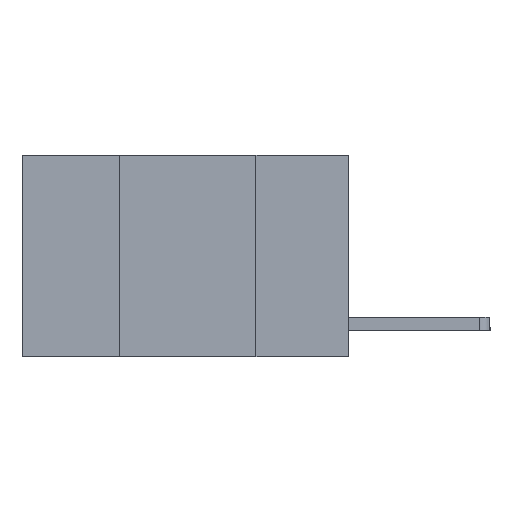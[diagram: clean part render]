
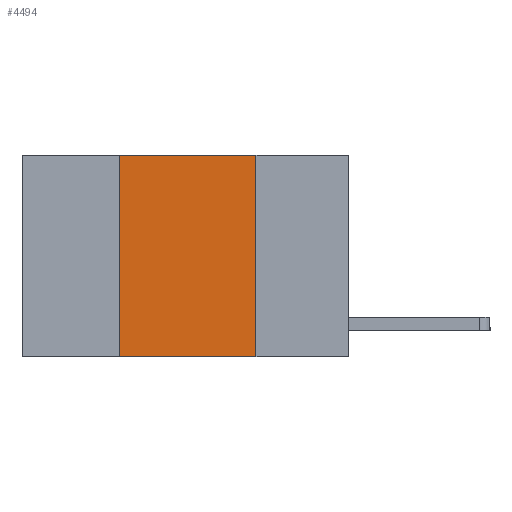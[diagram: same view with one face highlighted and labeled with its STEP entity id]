
A CAD part, left-side view. The second image highlights one B-rep face of the part: STEP entity #4494.
In plain terms, the highlighted planar face has unit normal (-1, 0, 0).
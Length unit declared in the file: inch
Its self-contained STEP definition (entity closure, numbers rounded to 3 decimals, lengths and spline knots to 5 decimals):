
#85 = CARTESIAN_POINT ( 'NONE',  ( 0., 0.17, 0. ) ) ;
#188 = DIRECTION ( 'NONE',  ( 0., -1., 0. ) ) ;
#245 = LINE ( 'NONE', #10368, #9955 ) ;
#270 = DIRECTION ( 'NONE',  ( 0., 0., 1. ) ) ;
#405 = PLANE ( 'NONE',  #7174 ) ;
#685 = ORIENTED_EDGE ( 'NONE', *, *, #8612, .T. ) ;
#690 = DIRECTION ( 'NONE',  ( 0., 0., -1. ) ) ;
#1046 = ORIENTED_EDGE ( 'NONE', *, *, #2373, .F. ) ;
#1174 = CARTESIAN_POINT ( 'NONE',  ( 0., 0.6, 0. ) ) ;
#1362 = ORIENTED_EDGE ( 'NONE', *, *, #2544, .F. ) ;
#1906 = EDGE_CURVE ( 'NONE', #4791, #5321, #5420, .T. ) ;
#2157 = CARTESIAN_POINT ( 'NONE',  ( 0., 0.17, -0.37 ) ) ;
#2373 = EDGE_CURVE ( 'NONE', #3136, #4791, #3015, .T. ) ;
#2544 = EDGE_CURVE ( 'NONE', #5321, #9673, #6558, .T. ) ;
#3015 = LINE ( 'NONE', #7922, #6894 ) ;
#3036 = DIRECTION ( 'NONE',  ( 1., 0., 0. ) ) ;
#3136 = VERTEX_POINT ( 'NONE', #5265 ) ;
#3418 = CARTESIAN_POINT ( 'NONE',  ( 0., 0.42, 0. ) ) ;
#3748 = DIRECTION ( 'NONE',  ( 0., -1., 0. ) ) ;
#3852 = VECTOR ( 'NONE', #3748, 39.37008 ) ;
#4494 = ADVANCED_FACE ( 'NONE', ( #7162 ), #405, .F. ) ;
#4699 = DIRECTION ( 'NONE',  ( 0., 0., -1. ) ) ;
#4791 = VERTEX_POINT ( 'NONE', #3418 ) ;
#4860 = EDGE_LOOP ( 'NONE', ( #1362, #9239, #1046, #685 ) ) ;
#5265 = CARTESIAN_POINT ( 'NONE',  ( 0., 0.42, -0.37 ) ) ;
#5321 = VERTEX_POINT ( 'NONE', #85 ) ;
#5420 = LINE ( 'NONE', #1174, #3852 ) ;
#6558 = LINE ( 'NONE', #9203, #7248 ) ;
#6894 = VECTOR ( 'NONE', #270, 39.37008 ) ;
#7162 = FACE_OUTER_BOUND ( 'NONE', #4860, .T. ) ;
#7174 = AXIS2_PLACEMENT_3D ( 'NONE', #9868, #3036, #4699 ) ;
#7248 = VECTOR ( 'NONE', #690, 39.37008 ) ;
#7922 = CARTESIAN_POINT ( 'NONE',  ( 0., 0.42, 0. ) ) ;
#8612 = EDGE_CURVE ( 'NONE', #3136, #9673, #245, .T. ) ;
#9203 = CARTESIAN_POINT ( 'NONE',  ( 0., 0.17, 0. ) ) ;
#9239 = ORIENTED_EDGE ( 'NONE', *, *, #1906, .F. ) ;
#9673 = VERTEX_POINT ( 'NONE', #2157 ) ;
#9868 = CARTESIAN_POINT ( 'NONE',  ( 0., 0.6, 0. ) ) ;
#9955 = VECTOR ( 'NONE', #188, 39.37008 ) ;
#10368 = CARTESIAN_POINT ( 'NONE',  ( 0., 0.6, -0.37 ) ) ;
